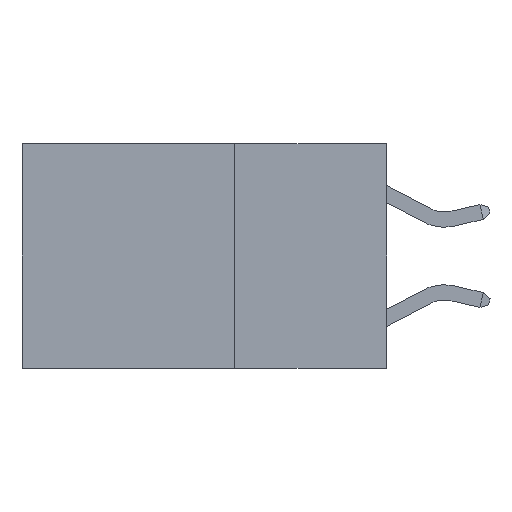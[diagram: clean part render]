
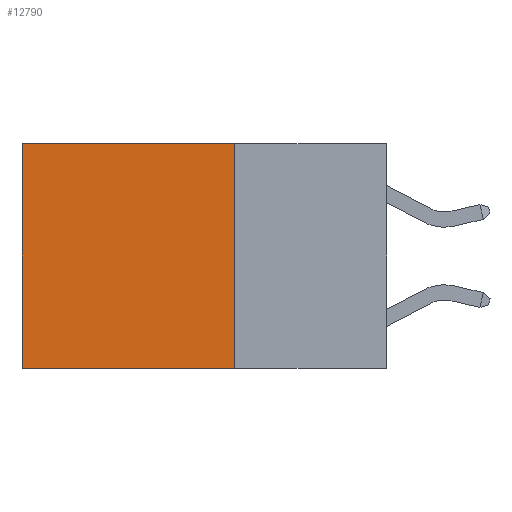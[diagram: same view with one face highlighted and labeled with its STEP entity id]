
A CAD part, left-side view. The second image highlights one B-rep face of the part: STEP entity #12790.
In plain terms, the highlighted planar face has unit normal (-1, 0, 0).
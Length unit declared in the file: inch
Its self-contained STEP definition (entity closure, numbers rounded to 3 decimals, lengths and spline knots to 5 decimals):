
#15 = LINE ( 'NONE', #9689, #5007 ) ;
#337 = CARTESIAN_POINT ( 'NONE',  ( 0.2625, 0.25, 0. ) ) ;
#1335 = CARTESIAN_POINT ( 'NONE',  ( 0.2625, 0.6, 0. ) ) ;
#1476 = EDGE_CURVE ( 'NONE', #26846, #27209, #15, .T. ) ;
#2164 = CARTESIAN_POINT ( 'NONE',  ( 0.2625, 0.6, -0.37 ) ) ;
#3143 = PLANE ( 'NONE',  #13563 ) ;
#3431 = DIRECTION ( 'NONE',  ( 0., 0., -1. ) ) ;
#3595 = LINE ( 'NONE', #25274, #9249 ) ;
#4299 = EDGE_CURVE ( 'NONE', #6172, #23836, #21427, .T. ) ;
#4615 = DIRECTION ( 'NONE',  ( 0., 1., 0. ) ) ;
#5007 = VECTOR ( 'NONE', #24456, 39.37008 ) ;
#5420 = VECTOR ( 'NONE', #4615, 39.37008 ) ;
#6172 = VERTEX_POINT ( 'NONE', #14735 ) ;
#6333 = EDGE_CURVE ( 'NONE', #26846, #6172, #16681, .T. ) ;
#6578 = ORIENTED_EDGE ( 'NONE', *, *, #8723, .F. ) ;
#7441 = DIRECTION ( 'NONE',  ( 1., 0., 0. ) ) ;
#8723 = EDGE_CURVE ( 'NONE', #27209, #23836, #3595, .T. ) ;
#8926 = CARTESIAN_POINT ( 'NONE',  ( 0.2625, 0.25, -0.37 ) ) ;
#9249 = VECTOR ( 'NONE', #10660, 39.37008 ) ;
#9689 = CARTESIAN_POINT ( 'NONE',  ( 0.2625, 0.25, 0. ) ) ;
#10660 = DIRECTION ( 'NONE',  ( 0., 1., 0. ) ) ;
#11888 = CARTESIAN_POINT ( 'NONE',  ( 0.2625, 0.25, 0. ) ) ;
#12790 = ADVANCED_FACE ( 'NONE', ( #21232 ), #3143, .F. ) ;
#13450 = ORIENTED_EDGE ( 'NONE', *, *, #1476, .F. ) ;
#13563 = AXIS2_PLACEMENT_3D ( 'NONE', #22122, #7441, #22214 ) ;
#14735 = CARTESIAN_POINT ( 'NONE',  ( 0.2625, 0.6, 0. ) ) ;
#16681 = LINE ( 'NONE', #337, #5420 ) ;
#17338 = ORIENTED_EDGE ( 'NONE', *, *, #6333, .T. ) ;
#17858 = EDGE_LOOP ( 'NONE', ( #20973, #6578, #13450, #17338 ) ) ;
#20750 = VECTOR ( 'NONE', #3431, 39.37008 ) ;
#20973 = ORIENTED_EDGE ( 'NONE', *, *, #4299, .T. ) ;
#21232 = FACE_OUTER_BOUND ( 'NONE', #17858, .T. ) ;
#21427 = LINE ( 'NONE', #1335, #20750 ) ;
#22122 = CARTESIAN_POINT ( 'NONE',  ( 0.2625, 0.25, 0. ) ) ;
#22214 = DIRECTION ( 'NONE',  ( 0., 0., -1. ) ) ;
#23836 = VERTEX_POINT ( 'NONE', #2164 ) ;
#24456 = DIRECTION ( 'NONE',  ( 0., 0., -1. ) ) ;
#25274 = CARTESIAN_POINT ( 'NONE',  ( 0.2625, 0.25, -0.37 ) ) ;
#26846 = VERTEX_POINT ( 'NONE', #11888 ) ;
#27209 = VERTEX_POINT ( 'NONE', #8926 ) ;
